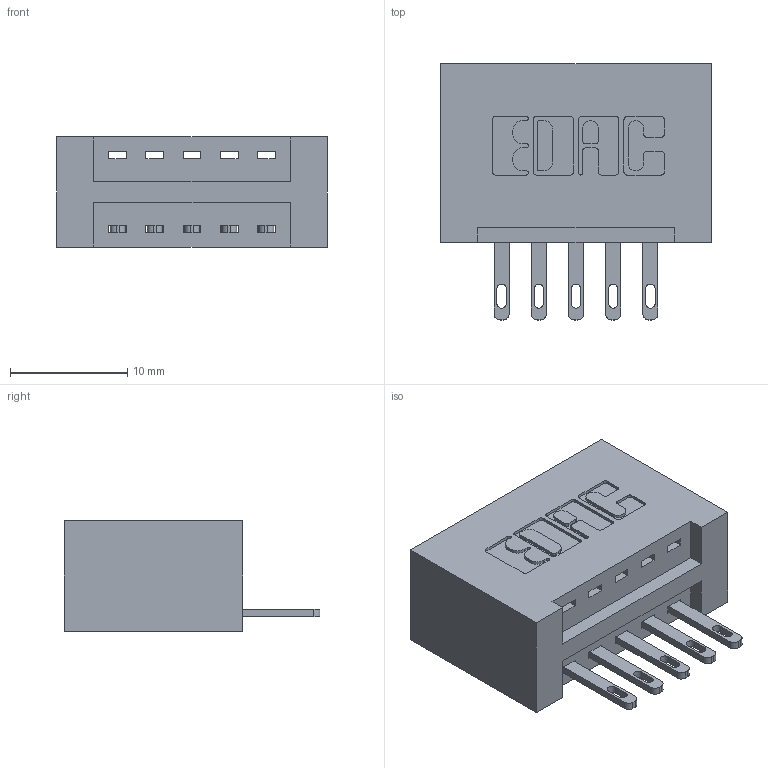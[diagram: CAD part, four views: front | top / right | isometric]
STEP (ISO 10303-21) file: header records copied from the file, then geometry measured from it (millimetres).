
FILE_DESCRIPTION (( 'STEP AP203' ), '1' );
FILE_NAME ('346-005-500-101.STEP', '2018-08-17T01:56:59', ( '' ), ( '' ), 'SwSTEP 2.0', 'SolidWorks 2016', '' );
FILE_SCHEMA (( 'CONFIG_CONTROL_DESIGN' ));
Length unit declared in the file: inch
Products named in the file (3): 346 Part_No Mounting Lugs; 345-292-001_345-293-100; 346-005-500-101
Assembly tree (6 placements, depth 2):
  346-005-500-101
    346 Part_No Mounting Lugs
    345-292-001_345-293-100  x5
Bounding box: 23.11 x 21.84 x 9.4 mm (x, y, z)
Volume: 2510.1 mm3; surface area: 2824.8 mm2
Topology: 6 solids, 6 shells, 384 faces, 1145 edges, 762 vertices
Faces by surface type: plane 242, cylinder 142
Entity records: 7737 total; most frequent: CARTESIAN_POINT 1343, ORIENTED_EDGE 1282, DIRECTION 1227, EDGE_CURVE 641, VECTOR 493, LINE 493, VERTEX_POINT 426, AXIS2_PLACEMENT_3D 367
